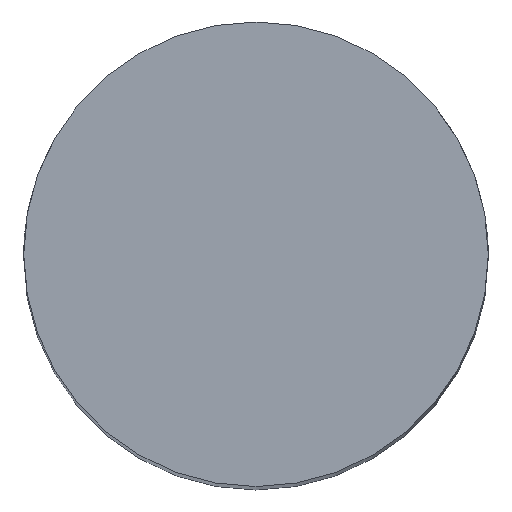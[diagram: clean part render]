
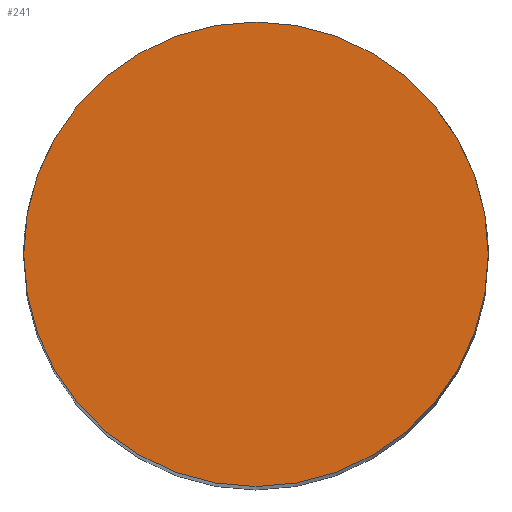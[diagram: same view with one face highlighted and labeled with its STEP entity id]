
A CAD part, top view. The second image highlights one B-rep face of the part: STEP entity #241.
In plain terms, the highlighted planar face has unit normal (0, 0, 1).
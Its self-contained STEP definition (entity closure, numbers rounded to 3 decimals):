
#83 = CIRCLE ( 'NONE', #436, 1.349 ) ;
#108 = CIRCLE ( 'NONE', #136, 1.349 ) ;
#136 = AXIS2_PLACEMENT_3D ( 'NONE', #406, #403, #401 ) ;
#147 = FACE_OUTER_BOUND ( 'NONE', #331, .T. ) ;
#157 = DIRECTION ( 'NONE',  ( 1., 0., 0. ) ) ;
#160 = AXIS2_PLACEMENT_3D ( 'NONE', #315, #359, #157 ) ;
#241 = ADVANCED_FACE ( 'NONE', ( #147 ), #400, .T. ) ;
#247 = DIRECTION ( 'NONE',  ( 1., 0., 0. ) ) ;
#251 = DIRECTION ( 'NONE',  ( 0., 0., -1. ) ) ;
#254 = ORIENTED_EDGE ( 'NONE', *, *, #297, .F. ) ;
#255 = CARTESIAN_POINT ( 'NONE',  ( 0., 0., 0. ) ) ;
#284 = CARTESIAN_POINT ( 'NONE',  ( 1.349, 0., 0. ) ) ;
#297 = EDGE_CURVE ( 'NONE', #419, #351, #108, .T. ) ;
#315 = CARTESIAN_POINT ( 'NONE',  ( 0., 0., 0. ) ) ;
#331 = EDGE_LOOP ( 'NONE', ( #254, #346 ) ) ;
#346 = ORIENTED_EDGE ( 'NONE', *, *, #407, .F. ) ;
#351 = VERTEX_POINT ( 'NONE', #364 ) ;
#359 = DIRECTION ( 'NONE',  ( 0., 0., 1. ) ) ;
#364 = CARTESIAN_POINT ( 'NONE',  ( -1.349, 0., 0. ) ) ;
#400 = PLANE ( 'NONE',  #160 ) ;
#401 = DIRECTION ( 'NONE',  ( 1., 0., 0. ) ) ;
#403 = DIRECTION ( 'NONE',  ( 0., 0., -1. ) ) ;
#406 = CARTESIAN_POINT ( 'NONE',  ( 0., 0., 0. ) ) ;
#407 = EDGE_CURVE ( 'NONE', #351, #419, #83, .T. ) ;
#419 = VERTEX_POINT ( 'NONE', #284 ) ;
#436 = AXIS2_PLACEMENT_3D ( 'NONE', #255, #251, #247 ) ;
